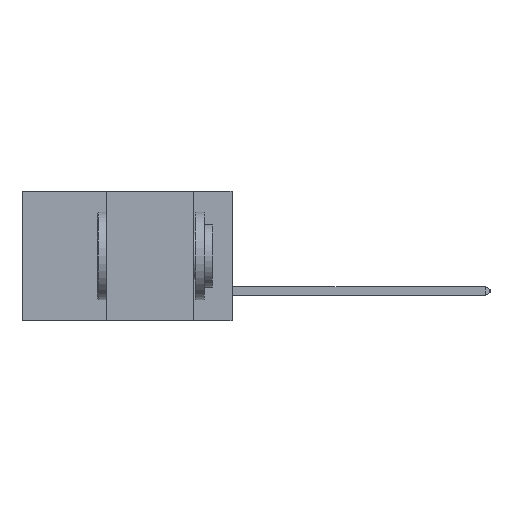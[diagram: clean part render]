
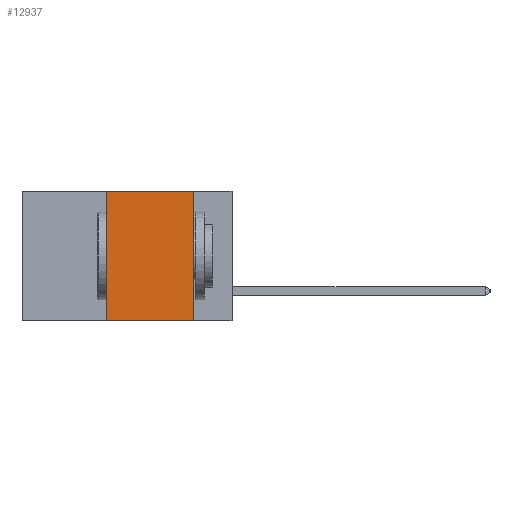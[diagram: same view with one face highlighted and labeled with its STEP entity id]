
A CAD part, left-side view. The second image highlights one B-rep face of the part: STEP entity #12937.
In plain terms, the highlighted planar face has unit normal (-1, 0, 0).
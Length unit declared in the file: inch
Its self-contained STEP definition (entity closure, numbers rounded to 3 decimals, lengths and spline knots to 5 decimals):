
#80 = EDGE_CURVE ( 'NONE', #5099, #13585, #10389, .T. ) ;
#427 = DIRECTION ( 'NONE',  ( 0., -1., 0. ) ) ;
#466 = CARTESIAN_POINT ( 'NONE',  ( 0., 0.6, -0.37 ) ) ;
#703 = EDGE_CURVE ( 'NONE', #1630, #5099, #13283, .T. ) ;
#888 = DIRECTION ( 'NONE',  ( 0., 0., -1. ) ) ;
#892 = DIRECTION ( 'NONE',  ( 0., -1., 0. ) ) ;
#1630 = VERTEX_POINT ( 'NONE', #6491 ) ;
#3342 = DIRECTION ( 'NONE',  ( 0., 0., -1. ) ) ;
#3368 = LINE ( 'NONE', #466, #8726 ) ;
#3831 = EDGE_LOOP ( 'NONE', ( #4579, #7620, #7932, #13458 ) ) ;
#4336 = PLANE ( 'NONE',  #9854 ) ;
#4579 = ORIENTED_EDGE ( 'NONE', *, *, #6380, .F. ) ;
#5099 = VERTEX_POINT ( 'NONE', #7828 ) ;
#5639 = CARTESIAN_POINT ( 'NONE',  ( 0., 0.6, 0. ) ) ;
#5793 = EDGE_CURVE ( 'NONE', #1630, #6151, #3368, .T. ) ;
#6151 = VERTEX_POINT ( 'NONE', #11081 ) ;
#6380 = EDGE_CURVE ( 'NONE', #13585, #6151, #10415, .T. ) ;
#6491 = CARTESIAN_POINT ( 'NONE',  ( 0., 0.36, -0.37 ) ) ;
#7482 = VECTOR ( 'NONE', #3342, 39.37008 ) ;
#7598 = DIRECTION ( 'NONE',  ( 1., 0., 0. ) ) ;
#7620 = ORIENTED_EDGE ( 'NONE', *, *, #80, .F. ) ;
#7828 = CARTESIAN_POINT ( 'NONE',  ( 0., 0.36, 0. ) ) ;
#7932 = ORIENTED_EDGE ( 'NONE', *, *, #703, .F. ) ;
#8051 = VECTOR ( 'NONE', #10677, 39.37008 ) ;
#8726 = VECTOR ( 'NONE', #427, 39.37008 ) ;
#9762 = VECTOR ( 'NONE', #892, 39.37008 ) ;
#9854 = AXIS2_PLACEMENT_3D ( 'NONE', #13469, #7598, #888 ) ;
#10389 = LINE ( 'NONE', #5639, #9762 ) ;
#10415 = LINE ( 'NONE', #12102, #7482 ) ;
#10677 = DIRECTION ( 'NONE',  ( 0., 0., 1. ) ) ;
#10742 = CARTESIAN_POINT ( 'NONE',  ( 0., 0.36, 0. ) ) ;
#11081 = CARTESIAN_POINT ( 'NONE',  ( 0., 0.11, -0.37 ) ) ;
#11357 = FACE_OUTER_BOUND ( 'NONE', #3831, .T. ) ;
#12102 = CARTESIAN_POINT ( 'NONE',  ( 0., 0.11, 0. ) ) ;
#12937 = ADVANCED_FACE ( 'NONE', ( #11357 ), #4336, .F. ) ;
#13283 = LINE ( 'NONE', #10742, #8051 ) ;
#13382 = CARTESIAN_POINT ( 'NONE',  ( 0., 0.11, 0. ) ) ;
#13458 = ORIENTED_EDGE ( 'NONE', *, *, #5793, .T. ) ;
#13469 = CARTESIAN_POINT ( 'NONE',  ( 0., 0.6, 0. ) ) ;
#13585 = VERTEX_POINT ( 'NONE', #13382 ) ;
